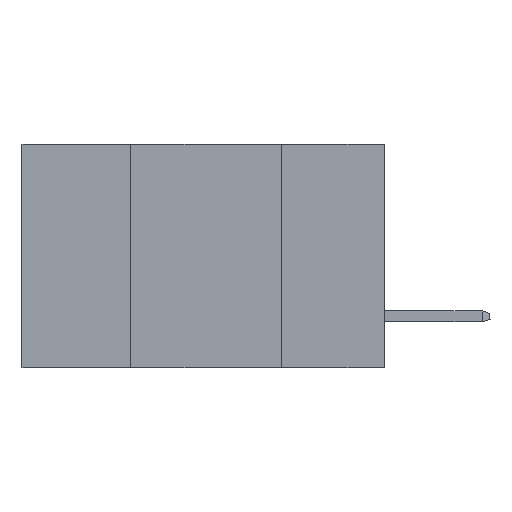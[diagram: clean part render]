
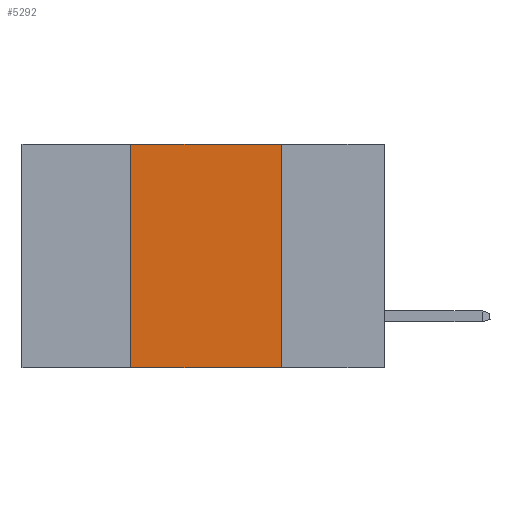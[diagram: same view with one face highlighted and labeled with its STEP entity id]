
A CAD part, left-side view. The second image highlights one B-rep face of the part: STEP entity #5292.
In plain terms, the highlighted planar face has unit normal (-1, 0, 0).
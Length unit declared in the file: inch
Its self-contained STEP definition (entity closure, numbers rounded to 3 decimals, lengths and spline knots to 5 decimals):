
#325 = DIRECTION ( 'NONE',  ( 0., 0., -1. ) ) ;
#1405 = VECTOR ( 'NONE', #3195, 39.37008 ) ;
#1719 = VERTEX_POINT ( 'NONE', #14152 ) ;
#1798 = LINE ( 'NONE', #3311, #1405 ) ;
#1864 = DIRECTION ( 'NONE',  ( 0., -1., 0. ) ) ;
#2427 = EDGE_CURVE ( 'NONE', #8698, #15801, #1798, .T. ) ;
#2449 = ORIENTED_EDGE ( 'NONE', *, *, #6611, .T. ) ;
#2553 = LINE ( 'NONE', #7904, #10902 ) ;
#3051 = CARTESIAN_POINT ( 'NONE',  ( 0., 0.17, 0. ) ) ;
#3195 = DIRECTION ( 'NONE',  ( 0., 0., -1. ) ) ;
#3311 = CARTESIAN_POINT ( 'NONE',  ( 0., 0.17, 0. ) ) ;
#3543 = VECTOR ( 'NONE', #9156, 39.37008 ) ;
#4306 = ORIENTED_EDGE ( 'NONE', *, *, #10051, .F. ) ;
#4482 = CARTESIAN_POINT ( 'NONE',  ( 0., 0.17, -0.37 ) ) ;
#4946 = CARTESIAN_POINT ( 'NONE',  ( 0., 0.42, 0. ) ) ;
#5234 = PLANE ( 'NONE',  #7667 ) ;
#5292 = ADVANCED_FACE ( 'NONE', ( #6294 ), #5234, .F. ) ;
#6294 = FACE_OUTER_BOUND ( 'NONE', #8114, .T. ) ;
#6611 = EDGE_CURVE ( 'NONE', #1719, #15801, #2553, .T. ) ;
#6679 = VECTOR ( 'NONE', #1864, 39.37008 ) ;
#6712 = CARTESIAN_POINT ( 'NONE',  ( 0., 0.6, 0. ) ) ;
#6893 = ORIENTED_EDGE ( 'NONE', *, *, #2427, .F. ) ;
#7667 = AXIS2_PLACEMENT_3D ( 'NONE', #7793, #13960, #325 ) ;
#7793 = CARTESIAN_POINT ( 'NONE',  ( 0., 0.6, 0. ) ) ;
#7904 = CARTESIAN_POINT ( 'NONE',  ( 0., 0.6, -0.37 ) ) ;
#8114 = EDGE_LOOP ( 'NONE', ( #6893, #14907, #4306, #2449 ) ) ;
#8659 = EDGE_CURVE ( 'NONE', #14816, #8698, #13434, .T. ) ;
#8698 = VERTEX_POINT ( 'NONE', #3051 ) ;
#9156 = DIRECTION ( 'NONE',  ( 0., 0., 1. ) ) ;
#10051 = EDGE_CURVE ( 'NONE', #1719, #14816, #13012, .T. ) ;
#10902 = VECTOR ( 'NONE', #15485, 39.37008 ) ;
#13012 = LINE ( 'NONE', #15330, #3543 ) ;
#13434 = LINE ( 'NONE', #6712, #6679 ) ;
#13960 = DIRECTION ( 'NONE',  ( 1., 0., 0. ) ) ;
#14152 = CARTESIAN_POINT ( 'NONE',  ( 0., 0.42, -0.37 ) ) ;
#14816 = VERTEX_POINT ( 'NONE', #4946 ) ;
#14907 = ORIENTED_EDGE ( 'NONE', *, *, #8659, .F. ) ;
#15330 = CARTESIAN_POINT ( 'NONE',  ( 0., 0.42, 0. ) ) ;
#15485 = DIRECTION ( 'NONE',  ( 0., -1., 0. ) ) ;
#15801 = VERTEX_POINT ( 'NONE', #4482 ) ;
